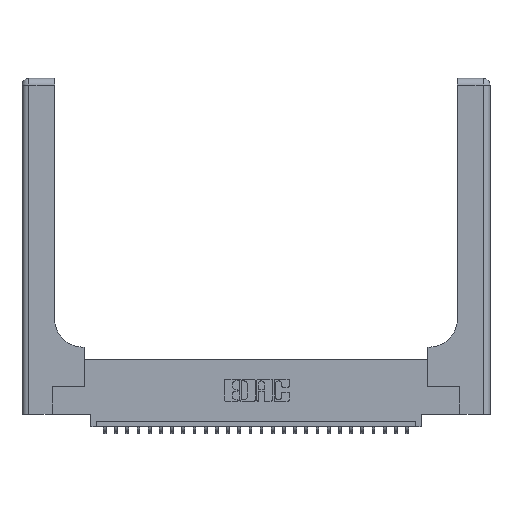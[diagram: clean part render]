
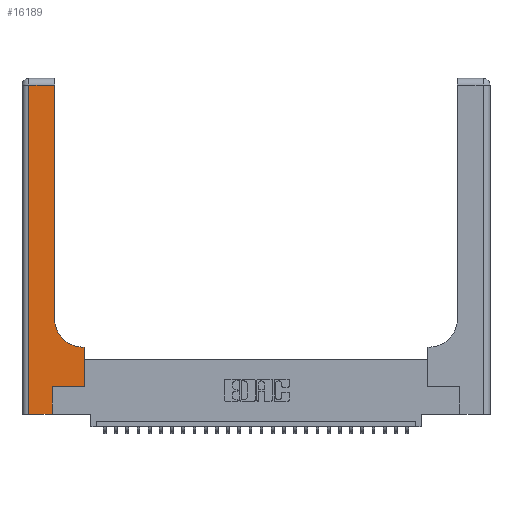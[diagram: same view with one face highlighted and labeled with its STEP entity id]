
A CAD part, top view. The second image highlights one B-rep face of the part: STEP entity #16189.
In plain terms, the highlighted planar face has unit normal (0, 0, 1).
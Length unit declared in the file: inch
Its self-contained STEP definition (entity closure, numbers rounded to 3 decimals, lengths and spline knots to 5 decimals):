
#226 = DIRECTION ( 'NONE',  ( 0., 0., -1. ) ) ;
#331 = VERTEX_POINT ( 'NONE', #3815 ) ;
#495 = VERTEX_POINT ( 'NONE', #8482 ) ;
#970 = CARTESIAN_POINT ( 'NONE',  ( 0.269, 0.25, 0.37 ) ) ;
#1210 = EDGE_CURVE ( 'NONE', #25558, #27471, #26690, .T. ) ;
#1241 = EDGE_CURVE ( 'NONE', #27471, #495, #26374, .T. ) ;
#1256 = VECTOR ( 'NONE', #27225, 39.37008 ) ;
#1443 = VECTOR ( 'NONE', #15744, 39.37008 ) ;
#1626 = CARTESIAN_POINT ( 'NONE',  ( 0.5585, 0.25, 0.37 ) ) ;
#2394 = VECTOR ( 'NONE', #14167, 39.37008 ) ;
#2718 = EDGE_CURVE ( 'NONE', #28368, #331, #12533, .T. ) ;
#2735 = ORIENTED_EDGE ( 'NONE', *, *, #19771, .T. ) ;
#2900 = CARTESIAN_POINT ( 'NONE',  ( 0.2915, 3., 0.37 ) ) ;
#3118 = CARTESIAN_POINT ( 'NONE',  ( 0.5415, 0.85, 0.37 ) ) ;
#3153 = VECTOR ( 'NONE', #23448, 39.37008 ) ;
#3639 = CARTESIAN_POINT ( 'NONE',  ( 0.2915, 0.6, 0.37 ) ) ;
#3815 = CARTESIAN_POINT ( 'NONE',  ( 0.06, 0., 0.37 ) ) ;
#4260 = VECTOR ( 'NONE', #5283, 39.37008 ) ;
#5060 = CARTESIAN_POINT ( 'NONE',  ( 0.269, 0., 0.37 ) ) ;
#5226 = VERTEX_POINT ( 'NONE', #970 ) ;
#5283 = DIRECTION ( 'NONE',  ( 1., 0., 0. ) ) ;
#5669 = AXIS2_PLACEMENT_3D ( 'NONE', #3118, #20860, #20768 ) ;
#7611 = EDGE_CURVE ( 'NONE', #27662, #9932, #13273, .T. ) ;
#7971 = ORIENTED_EDGE ( 'NONE', *, *, #1210, .T. ) ;
#8215 = CARTESIAN_POINT ( 'NONE',  ( 0.06, 3., 0.37 ) ) ;
#8482 = CARTESIAN_POINT ( 'NONE',  ( 0.5415, 0.6, 0.37 ) ) ;
#9008 = LINE ( 'NONE', #27912, #3153 ) ;
#9932 = VERTEX_POINT ( 'NONE', #16337 ) ;
#9953 = ORIENTED_EDGE ( 'NONE', *, *, #18898, .T. ) ;
#10990 = CIRCLE ( 'NONE', #5669, 0.25 ) ;
#11127 = CARTESIAN_POINT ( 'NONE',  ( 0.5585, 0.6, 0.37 ) ) ;
#11311 = CARTESIAN_POINT ( 'NONE',  ( 0.269, 0., 0.37 ) ) ;
#12308 = VECTOR ( 'NONE', #19184, 39.37008 ) ;
#12533 = LINE ( 'NONE', #8215, #14585 ) ;
#12645 = DIRECTION ( 'NONE',  ( 0., 1., 0. ) ) ;
#13273 = LINE ( 'NONE', #2900, #1256 ) ;
#14167 = DIRECTION ( 'NONE',  ( 1., 0., 0. ) ) ;
#14585 = VECTOR ( 'NONE', #14815, 39.37008 ) ;
#14653 = CARTESIAN_POINT ( 'NONE',  ( 0.2915, 0.85, 0.37 ) ) ;
#14815 = DIRECTION ( 'NONE',  ( 0., -1., 0. ) ) ;
#14879 = ORIENTED_EDGE ( 'NONE', *, *, #1241, .T. ) ;
#15662 = PLANE ( 'NONE',  #20319 ) ;
#15744 = DIRECTION ( 'NONE',  ( 0., 1., 0. ) ) ;
#16189 = ADVANCED_FACE ( 'NONE', ( #25869 ), #15662, .F. ) ;
#16337 = CARTESIAN_POINT ( 'NONE',  ( 0.2915, 2.94, 0.37 ) ) ;
#17235 = LINE ( 'NONE', #11311, #1443 ) ;
#17650 = LINE ( 'NONE', #18416, #4260 ) ;
#17711 = EDGE_CURVE ( 'NONE', #27499, #5226, #17235, .T. ) ;
#17826 = VECTOR ( 'NONE', #12645, 39.37008 ) ;
#18416 = CARTESIAN_POINT ( 'NONE',  ( 0., 0., 0.37 ) ) ;
#18651 = EDGE_LOOP ( 'NONE', ( #27295, #21381, #26056, #26102, #21291, #2735, #7971, #14879, #9953 ) ) ;
#18898 = EDGE_CURVE ( 'NONE', #495, #27662, #10990, .T. ) ;
#19063 = CARTESIAN_POINT ( 'NONE',  ( 0.06, 2.94, 0.37 ) ) ;
#19184 = DIRECTION ( 'NONE',  ( -1., 0., 0. ) ) ;
#19771 = EDGE_CURVE ( 'NONE', #5226, #25558, #22957, .T. ) ;
#20319 = AXIS2_PLACEMENT_3D ( 'NONE', #24446, #226, #26351 ) ;
#20768 = DIRECTION ( 'NONE',  ( 1., 0., 0. ) ) ;
#20860 = DIRECTION ( 'NONE',  ( 0., 0., -1. ) ) ;
#21291 = ORIENTED_EDGE ( 'NONE', *, *, #17711, .T. ) ;
#21381 = ORIENTED_EDGE ( 'NONE', *, *, #25190, .T. ) ;
#21968 = EDGE_CURVE ( 'NONE', #331, #27499, #17650, .T. ) ;
#22888 = CARTESIAN_POINT ( 'NONE',  ( 0.269, 0.25, 0.37 ) ) ;
#22957 = LINE ( 'NONE', #22888, #2394 ) ;
#23448 = DIRECTION ( 'NONE',  ( -1., 0., 0. ) ) ;
#24446 = CARTESIAN_POINT ( 'NONE',  ( 0., 3., 0.37 ) ) ;
#25190 = EDGE_CURVE ( 'NONE', #9932, #28368, #9008, .T. ) ;
#25558 = VERTEX_POINT ( 'NONE', #25639 ) ;
#25639 = CARTESIAN_POINT ( 'NONE',  ( 0.5585, 0.25, 0.37 ) ) ;
#25869 = FACE_OUTER_BOUND ( 'NONE', #18651, .T. ) ;
#26056 = ORIENTED_EDGE ( 'NONE', *, *, #2718, .T. ) ;
#26102 = ORIENTED_EDGE ( 'NONE', *, *, #21968, .T. ) ;
#26351 = DIRECTION ( 'NONE',  ( -1., 0., 0. ) ) ;
#26374 = LINE ( 'NONE', #3639, #12308 ) ;
#26690 = LINE ( 'NONE', #1626, #17826 ) ;
#27225 = DIRECTION ( 'NONE',  ( 0., 1., 0. ) ) ;
#27295 = ORIENTED_EDGE ( 'NONE', *, *, #7611, .T. ) ;
#27471 = VERTEX_POINT ( 'NONE', #11127 ) ;
#27499 = VERTEX_POINT ( 'NONE', #5060 ) ;
#27662 = VERTEX_POINT ( 'NONE', #14653 ) ;
#27912 = CARTESIAN_POINT ( 'NONE',  ( 0., 2.94, 0.37 ) ) ;
#28368 = VERTEX_POINT ( 'NONE', #19063 ) ;
